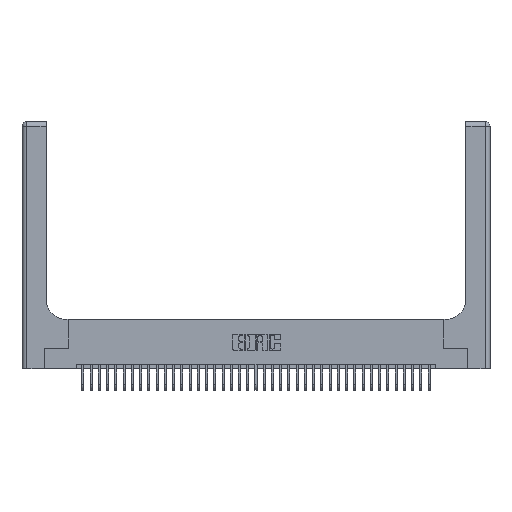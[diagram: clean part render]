
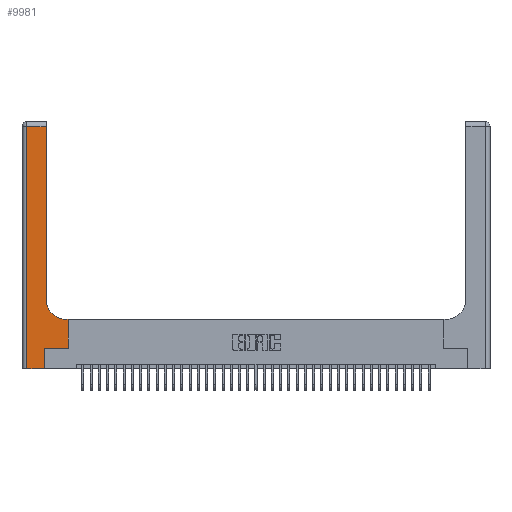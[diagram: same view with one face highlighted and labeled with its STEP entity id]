
A CAD part, top view. The second image highlights one B-rep face of the part: STEP entity #9981.
In plain terms, the highlighted planar face has unit normal (0, 0, 1).
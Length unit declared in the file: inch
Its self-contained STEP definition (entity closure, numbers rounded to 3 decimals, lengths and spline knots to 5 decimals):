
#450 = ORIENTED_EDGE ( 'NONE', *, *, #19271, .T. ) ;
#460 = CARTESIAN_POINT ( 'NONE',  ( 0.269, 0.25, 0.37 ) ) ;
#1177 = CARTESIAN_POINT ( 'NONE',  ( 0.2915, 0.6, 0.37 ) ) ;
#2611 = VERTEX_POINT ( 'NONE', #30771 ) ;
#3115 = CARTESIAN_POINT ( 'NONE',  ( 0.269, 0., 0.37 ) ) ;
#4536 = LINE ( 'NONE', #37011, #28459 ) ;
#5905 = CARTESIAN_POINT ( 'NONE',  ( 0.06, 3., 0.37 ) ) ;
#6225 = EDGE_CURVE ( 'NONE', #14861, #25922, #35883, .T. ) ;
#6907 = VECTOR ( 'NONE', #30491, 39.37008 ) ;
#7326 = DIRECTION ( 'NONE',  ( -1., 0., 0. ) ) ;
#7813 = LINE ( 'NONE', #5905, #17527 ) ;
#8686 = EDGE_LOOP ( 'NONE', ( #29052, #20755, #29912, #15674, #450, #20834, #16789, #27598, #31284 ) ) ;
#9060 = DIRECTION ( 'NONE',  ( 0., 1., 0. ) ) ;
#9469 = CARTESIAN_POINT ( 'NONE',  ( 0.5585, 0.25, 0.37 ) ) ;
#9620 = VECTOR ( 'NONE', #24938, 39.37008 ) ;
#9886 = DIRECTION ( 'NONE',  ( 0., 1., 0. ) ) ;
#9981 = ADVANCED_FACE ( 'NONE', ( #20796 ), #39165, .F. ) ;
#10391 = VECTOR ( 'NONE', #9886, 39.37008 ) ;
#11022 = CARTESIAN_POINT ( 'NONE',  ( 0., 0., 0.37 ) ) ;
#11185 = VERTEX_POINT ( 'NONE', #30547 ) ;
#12025 = VERTEX_POINT ( 'NONE', #31255 ) ;
#12516 = CARTESIAN_POINT ( 'NONE',  ( 0.5585, 0.25, 0.37 ) ) ;
#14390 = VECTOR ( 'NONE', #9060, 39.37008 ) ;
#14595 = CARTESIAN_POINT ( 'NONE',  ( 0.2915, 0.85, 0.37 ) ) ;
#14861 = VERTEX_POINT ( 'NONE', #14595 ) ;
#15282 = AXIS2_PLACEMENT_3D ( 'NONE', #21178, #21593, #19125 ) ;
#15666 = CARTESIAN_POINT ( 'NONE',  ( 0.06, 0., 0.37 ) ) ;
#15674 = ORIENTED_EDGE ( 'NONE', *, *, #29973, .T. ) ;
#16789 = ORIENTED_EDGE ( 'NONE', *, *, #38996, .T. ) ;
#17527 = VECTOR ( 'NONE', #37236, 39.37008 ) ;
#19125 = DIRECTION ( 'NONE',  ( 1., 0., 0. ) ) ;
#19271 = EDGE_CURVE ( 'NONE', #12025, #37117, #40456, .T. ) ;
#20755 = ORIENTED_EDGE ( 'NONE', *, *, #22782, .T. ) ;
#20796 = FACE_OUTER_BOUND ( 'NONE', #8686, .T. ) ;
#20834 = ORIENTED_EDGE ( 'NONE', *, *, #23490, .T. ) ;
#21178 = CARTESIAN_POINT ( 'NONE',  ( 0.5415, 0.85, 0.37 ) ) ;
#21593 = DIRECTION ( 'NONE',  ( 0., 0., -1. ) ) ;
#21928 = VERTEX_POINT ( 'NONE', #12516 ) ;
#22424 = VERTEX_POINT ( 'NONE', #15666 ) ;
#22651 = LINE ( 'NONE', #9469, #14390 ) ;
#22782 = EDGE_CURVE ( 'NONE', #25922, #23736, #4536, .T. ) ;
#23490 = EDGE_CURVE ( 'NONE', #37117, #21928, #28878, .T. ) ;
#23736 = VERTEX_POINT ( 'NONE', #31858 ) ;
#23852 = VECTOR ( 'NONE', #29826, 39.37008 ) ;
#23860 = CIRCLE ( 'NONE', #15282, 0.25 ) ;
#24938 = DIRECTION ( 'NONE',  ( 0., 1., 0. ) ) ;
#25922 = VERTEX_POINT ( 'NONE', #39316 ) ;
#26870 = EDGE_CURVE ( 'NONE', #11185, #14861, #23860, .T. ) ;
#27084 = CARTESIAN_POINT ( 'NONE',  ( 0.269, 0.25, 0.37 ) ) ;
#27469 = EDGE_CURVE ( 'NONE', #23736, #22424, #7813, .T. ) ;
#27521 = DIRECTION ( 'NONE',  ( -1., 0., 0. ) ) ;
#27598 = ORIENTED_EDGE ( 'NONE', *, *, #32290, .T. ) ;
#28459 = VECTOR ( 'NONE', #34230, 39.37008 ) ;
#28878 = LINE ( 'NONE', #27084, #6907 ) ;
#29052 = ORIENTED_EDGE ( 'NONE', *, *, #6225, .T. ) ;
#29826 = DIRECTION ( 'NONE',  ( 1., 0., 0. ) ) ;
#29912 = ORIENTED_EDGE ( 'NONE', *, *, #27469, .T. ) ;
#29973 = EDGE_CURVE ( 'NONE', #22424, #12025, #37639, .T. ) ;
#30491 = DIRECTION ( 'NONE',  ( 1., 0., 0. ) ) ;
#30547 = CARTESIAN_POINT ( 'NONE',  ( 0.5415, 0.6, 0.37 ) ) ;
#30771 = CARTESIAN_POINT ( 'NONE',  ( 0.5585, 0.6, 0.37 ) ) ;
#31255 = CARTESIAN_POINT ( 'NONE',  ( 0.269, 0., 0.37 ) ) ;
#31284 = ORIENTED_EDGE ( 'NONE', *, *, #26870, .T. ) ;
#31858 = CARTESIAN_POINT ( 'NONE',  ( 0.06, 2.94, 0.37 ) ) ;
#32290 = EDGE_CURVE ( 'NONE', #2611, #11185, #40271, .T. ) ;
#32465 = VECTOR ( 'NONE', #7326, 39.37008 ) ;
#34230 = DIRECTION ( 'NONE',  ( -1., 0., 0. ) ) ;
#34932 = CARTESIAN_POINT ( 'NONE',  ( 0.2915, 3., 0.37 ) ) ;
#35883 = LINE ( 'NONE', #34932, #10391 ) ;
#36257 = AXIS2_PLACEMENT_3D ( 'NONE', #39304, #39435, #27521 ) ;
#37011 = CARTESIAN_POINT ( 'NONE',  ( 0., 2.94, 0.37 ) ) ;
#37117 = VERTEX_POINT ( 'NONE', #460 ) ;
#37236 = DIRECTION ( 'NONE',  ( 0., -1., 0. ) ) ;
#37639 = LINE ( 'NONE', #11022, #23852 ) ;
#38996 = EDGE_CURVE ( 'NONE', #21928, #2611, #22651, .T. ) ;
#39165 = PLANE ( 'NONE',  #36257 ) ;
#39304 = CARTESIAN_POINT ( 'NONE',  ( 0., 3., 0.37 ) ) ;
#39316 = CARTESIAN_POINT ( 'NONE',  ( 0.2915, 2.94, 0.37 ) ) ;
#39435 = DIRECTION ( 'NONE',  ( 0., 0., -1. ) ) ;
#40271 = LINE ( 'NONE', #1177, #32465 ) ;
#40456 = LINE ( 'NONE', #3115, #9620 ) ;
